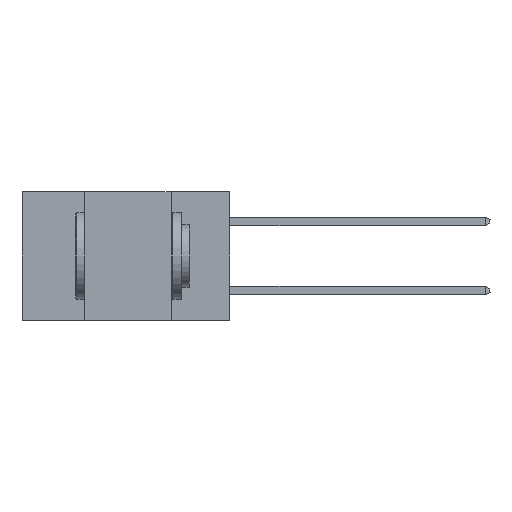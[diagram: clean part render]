
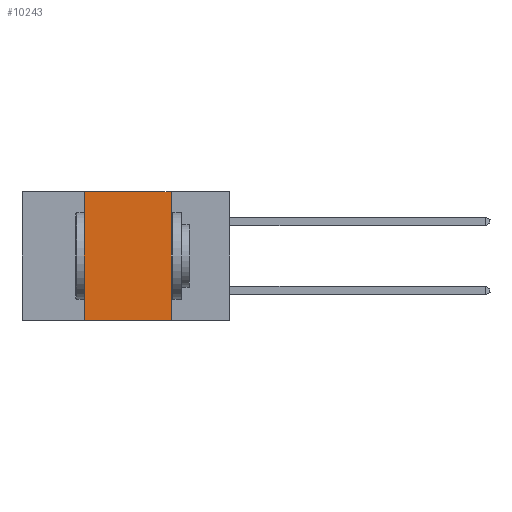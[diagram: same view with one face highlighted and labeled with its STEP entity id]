
A CAD part, left-side view. The second image highlights one B-rep face of the part: STEP entity #10243.
In plain terms, the highlighted planar face has unit normal (-1, 0, 0).
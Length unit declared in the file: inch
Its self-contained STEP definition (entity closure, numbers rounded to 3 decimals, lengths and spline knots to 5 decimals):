
#434 = EDGE_CURVE ( 'NONE', #31367, #17517, #1354, .T. ) ;
#1354 = LINE ( 'NONE', #2343, #6068 ) ;
#1589 = VECTOR ( 'NONE', #15325, 39.37008 ) ;
#2343 = CARTESIAN_POINT ( 'NONE',  ( 0., 0.6, 0. ) ) ;
#3492 = PLANE ( 'NONE',  #18062 ) ;
#5161 = LINE ( 'NONE', #10281, #1589 ) ;
#5925 = CARTESIAN_POINT ( 'NONE',  ( 0., 0.6, 0. ) ) ;
#6068 = VECTOR ( 'NONE', #22498, 39.37008 ) ;
#6689 = ORIENTED_EDGE ( 'NONE', *, *, #13524, .F. ) ;
#7806 = VECTOR ( 'NONE', #27374, 39.37008 ) ;
#7872 = LINE ( 'NONE', #10976, #13374 ) ;
#9001 = ORIENTED_EDGE ( 'NONE', *, *, #26863, .F. ) ;
#10243 = ADVANCED_FACE ( 'NONE', ( #31643 ), #3492, .F. ) ;
#10281 = CARTESIAN_POINT ( 'NONE',  ( 0., 0.6, -0.37 ) ) ;
#10976 = CARTESIAN_POINT ( 'NONE',  ( 0., 0.42, 0. ) ) ;
#11473 = CARTESIAN_POINT ( 'NONE',  ( 0., 0.17, -0.37 ) ) ;
#13374 = VECTOR ( 'NONE', #27310, 39.37008 ) ;
#13524 = EDGE_CURVE ( 'NONE', #16717, #31367, #7872, .T. ) ;
#14963 = EDGE_LOOP ( 'NONE', ( #9001, #31148, #6689, #22766 ) ) ;
#15325 = DIRECTION ( 'NONE',  ( 0., -1., 0. ) ) ;
#16717 = VERTEX_POINT ( 'NONE', #32350 ) ;
#17230 = LINE ( 'NONE', #27586, #7806 ) ;
#17517 = VERTEX_POINT ( 'NONE', #20917 ) ;
#18062 = AXIS2_PLACEMENT_3D ( 'NONE', #5925, #21096, #20880 ) ;
#20880 = DIRECTION ( 'NONE',  ( 0., 0., -1. ) ) ;
#20917 = CARTESIAN_POINT ( 'NONE',  ( 0., 0.17, 0. ) ) ;
#20943 = CARTESIAN_POINT ( 'NONE',  ( 0., 0.42, 0. ) ) ;
#21030 = EDGE_CURVE ( 'NONE', #16717, #21993, #5161, .T. ) ;
#21096 = DIRECTION ( 'NONE',  ( 1., 0., 0. ) ) ;
#21993 = VERTEX_POINT ( 'NONE', #11473 ) ;
#22498 = DIRECTION ( 'NONE',  ( 0., -1., 0. ) ) ;
#22766 = ORIENTED_EDGE ( 'NONE', *, *, #21030, .T. ) ;
#26863 = EDGE_CURVE ( 'NONE', #17517, #21993, #17230, .T. ) ;
#27310 = DIRECTION ( 'NONE',  ( 0., 0., 1. ) ) ;
#27374 = DIRECTION ( 'NONE',  ( 0., 0., -1. ) ) ;
#27586 = CARTESIAN_POINT ( 'NONE',  ( 0., 0.17, 0. ) ) ;
#31148 = ORIENTED_EDGE ( 'NONE', *, *, #434, .F. ) ;
#31367 = VERTEX_POINT ( 'NONE', #20943 ) ;
#31643 = FACE_OUTER_BOUND ( 'NONE', #14963, .T. ) ;
#32350 = CARTESIAN_POINT ( 'NONE',  ( 0., 0.42, -0.37 ) ) ;
